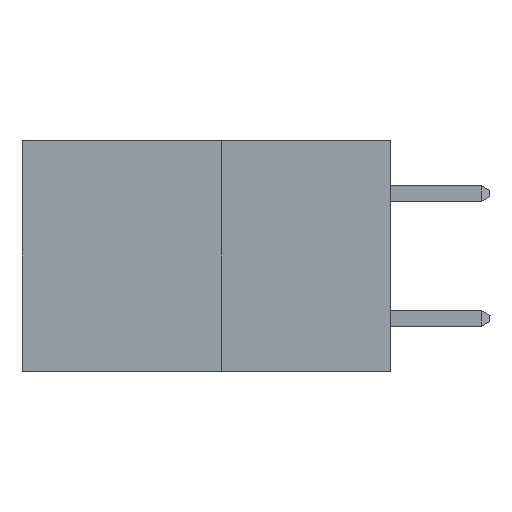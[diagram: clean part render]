
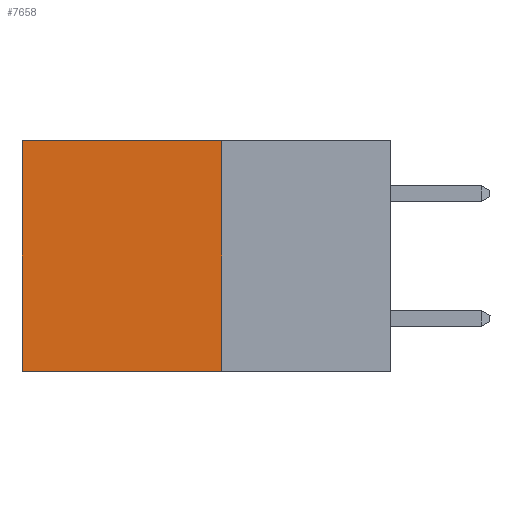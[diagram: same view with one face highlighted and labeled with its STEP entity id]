
A CAD part, left-side view. The second image highlights one B-rep face of the part: STEP entity #7658.
In plain terms, the highlighted planar face has unit normal (-1, 0, 0).
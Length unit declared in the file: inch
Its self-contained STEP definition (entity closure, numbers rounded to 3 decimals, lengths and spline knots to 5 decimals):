
#79 = CARTESIAN_POINT ( 'NONE',  ( 0.277, 0.27, 0. ) ) ;
#376 = DIRECTION ( 'NONE',  ( 0., 1., 0. ) ) ;
#638 = EDGE_CURVE ( 'NONE', #4452, #9914, #8642, .T. ) ;
#684 = CARTESIAN_POINT ( 'NONE',  ( 0.277, 0.27, -0.37 ) ) ;
#753 = EDGE_CURVE ( 'NONE', #9914, #4201, #7763, .T. ) ;
#1479 = DIRECTION ( 'NONE',  ( 0., 0., -1. ) ) ;
#1518 = DIRECTION ( 'NONE',  ( 0., 1., 0. ) ) ;
#1627 = CARTESIAN_POINT ( 'NONE',  ( 0.277, 0.59, -0.37 ) ) ;
#1650 = CARTESIAN_POINT ( 'NONE',  ( 0.277, 0.27, -0.37 ) ) ;
#1771 = DIRECTION ( 'NONE',  ( 0., 0., -1. ) ) ;
#1932 = CARTESIAN_POINT ( 'NONE',  ( 0.277, 0.27, 0. ) ) ;
#2370 = EDGE_LOOP ( 'NONE', ( #9656, #7791, #6278, #4027 ) ) ;
#2642 = LINE ( 'NONE', #3465, #4566 ) ;
#2866 = EDGE_CURVE ( 'NONE', #3399, #4201, #7954, .T. ) ;
#2938 = CARTESIAN_POINT ( 'NONE',  ( 0.277, 0.59, -0.37 ) ) ;
#3399 = VERTEX_POINT ( 'NONE', #1650 ) ;
#3425 = DIRECTION ( 'NONE',  ( 0., 0., -1. ) ) ;
#3465 = CARTESIAN_POINT ( 'NONE',  ( 0.277, 0.27, -0.37 ) ) ;
#3722 = EDGE_CURVE ( 'NONE', #4452, #3399, #2642, .T. ) ;
#4027 = ORIENTED_EDGE ( 'NONE', *, *, #638, .T. ) ;
#4201 = VERTEX_POINT ( 'NONE', #2938 ) ;
#4244 = CARTESIAN_POINT ( 'NONE',  ( 0.277, 0.27, -0.37 ) ) ;
#4452 = VERTEX_POINT ( 'NONE', #1932 ) ;
#4566 = VECTOR ( 'NONE', #3425, 39.37008 ) ;
#5958 = AXIS2_PLACEMENT_3D ( 'NONE', #684, #6251, #1479 ) ;
#6251 = DIRECTION ( 'NONE',  ( 1., 0., 0. ) ) ;
#6278 = ORIENTED_EDGE ( 'NONE', *, *, #3722, .F. ) ;
#7449 = CARTESIAN_POINT ( 'NONE',  ( 0.277, 0.59, 0. ) ) ;
#7548 = VECTOR ( 'NONE', #1771, 39.37008 ) ;
#7658 = ADVANCED_FACE ( 'NONE', ( #9545 ), #9832, .F. ) ;
#7763 = LINE ( 'NONE', #1627, #7548 ) ;
#7791 = ORIENTED_EDGE ( 'NONE', *, *, #2866, .F. ) ;
#7954 = LINE ( 'NONE', #4244, #9806 ) ;
#8418 = VECTOR ( 'NONE', #376, 39.37008 ) ;
#8642 = LINE ( 'NONE', #79, #8418 ) ;
#9545 = FACE_OUTER_BOUND ( 'NONE', #2370, .T. ) ;
#9656 = ORIENTED_EDGE ( 'NONE', *, *, #753, .T. ) ;
#9806 = VECTOR ( 'NONE', #1518, 39.37008 ) ;
#9832 = PLANE ( 'NONE',  #5958 ) ;
#9914 = VERTEX_POINT ( 'NONE', #7449 ) ;
